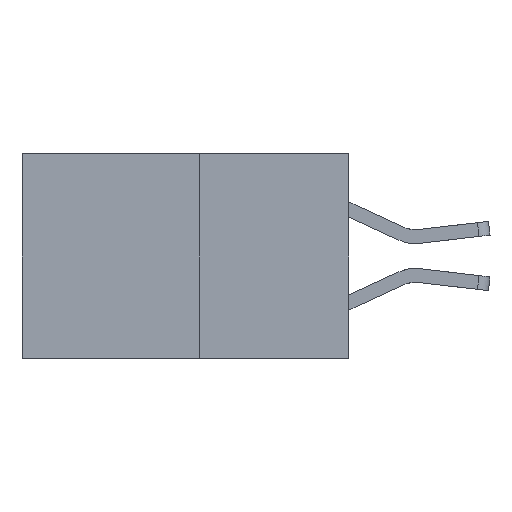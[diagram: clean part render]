
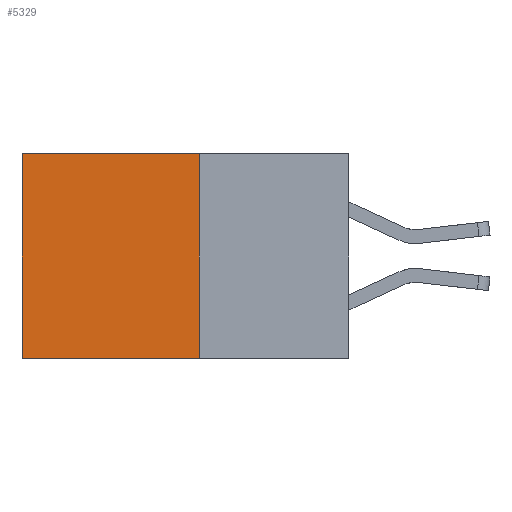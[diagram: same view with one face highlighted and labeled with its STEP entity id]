
A CAD part, left-side view. The second image highlights one B-rep face of the part: STEP entity #5329.
In plain terms, the highlighted planar face has unit normal (-1, 0, 0).
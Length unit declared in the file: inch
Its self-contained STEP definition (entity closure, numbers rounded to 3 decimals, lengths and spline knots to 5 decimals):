
#1139 = ORIENTED_EDGE ( 'NONE', *, *, #2398, .T. ) ;
#1299 = LINE ( 'NONE', #7399, #5611 ) ;
#1342 = CARTESIAN_POINT ( 'NONE',  ( 0.277, 0.27, 0. ) ) ;
#1524 = CARTESIAN_POINT ( 'NONE',  ( 0.277, 0.59, 0. ) ) ;
#1965 = EDGE_CURVE ( 'NONE', #7085, #8625, #1299, .T. ) ;
#2274 = AXIS2_PLACEMENT_3D ( 'NONE', #5498, #6585, #4598 ) ;
#2398 = EDGE_CURVE ( 'NONE', #8625, #8815, #10634, .T. ) ;
#2711 = CARTESIAN_POINT ( 'NONE',  ( 0.277, 0.59, -0.37 ) ) ;
#3270 = VECTOR ( 'NONE', #6212, 39.37008 ) ;
#3368 = CARTESIAN_POINT ( 'NONE',  ( 0.277, 0.27, -0.37 ) ) ;
#3403 = ORIENTED_EDGE ( 'NONE', *, *, #7781, .F. ) ;
#3440 = FACE_OUTER_BOUND ( 'NONE', #4851, .T. ) ;
#3569 = VECTOR ( 'NONE', #7149, 39.37008 ) ;
#4086 = LINE ( 'NONE', #7921, #10375 ) ;
#4598 = DIRECTION ( 'NONE',  ( 0., 0., -1. ) ) ;
#4851 = EDGE_LOOP ( 'NONE', ( #1139, #5229, #3403, #6484 ) ) ;
#5229 = ORIENTED_EDGE ( 'NONE', *, *, #6643, .F. ) ;
#5329 = ADVANCED_FACE ( 'NONE', ( #3440 ), #6513, .F. ) ;
#5498 = CARTESIAN_POINT ( 'NONE',  ( 0.277, 0.27, -0.37 ) ) ;
#5611 = VECTOR ( 'NONE', #10702, 39.37008 ) ;
#6212 = DIRECTION ( 'NONE',  ( 0., 0., -1. ) ) ;
#6484 = ORIENTED_EDGE ( 'NONE', *, *, #1965, .T. ) ;
#6513 = PLANE ( 'NONE',  #2274 ) ;
#6585 = DIRECTION ( 'NONE',  ( 1., 0., 0. ) ) ;
#6643 = EDGE_CURVE ( 'NONE', #10666, #8815, #4086, .T. ) ;
#6982 = CARTESIAN_POINT ( 'NONE',  ( 0.277, 0.27, -0.37 ) ) ;
#7085 = VERTEX_POINT ( 'NONE', #1342 ) ;
#7149 = DIRECTION ( 'NONE',  ( 0., 0., -1. ) ) ;
#7269 = CARTESIAN_POINT ( 'NONE',  ( 0.277, 0.59, -0.37 ) ) ;
#7399 = CARTESIAN_POINT ( 'NONE',  ( 0.277, 0.27, 0. ) ) ;
#7771 = DIRECTION ( 'NONE',  ( 0., 1., 0. ) ) ;
#7781 = EDGE_CURVE ( 'NONE', #7085, #10666, #7829, .T. ) ;
#7829 = LINE ( 'NONE', #6982, #3270 ) ;
#7921 = CARTESIAN_POINT ( 'NONE',  ( 0.277, 0.27, -0.37 ) ) ;
#8625 = VERTEX_POINT ( 'NONE', #1524 ) ;
#8815 = VERTEX_POINT ( 'NONE', #2711 ) ;
#10375 = VECTOR ( 'NONE', #7771, 39.37008 ) ;
#10634 = LINE ( 'NONE', #7269, #3569 ) ;
#10666 = VERTEX_POINT ( 'NONE', #3368 ) ;
#10702 = DIRECTION ( 'NONE',  ( 0., 1., 0. ) ) ;
